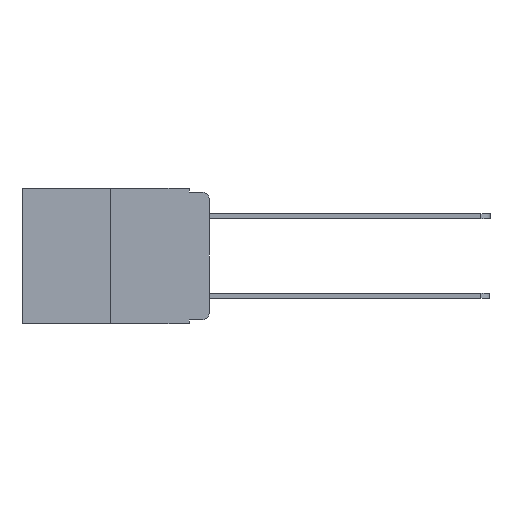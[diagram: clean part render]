
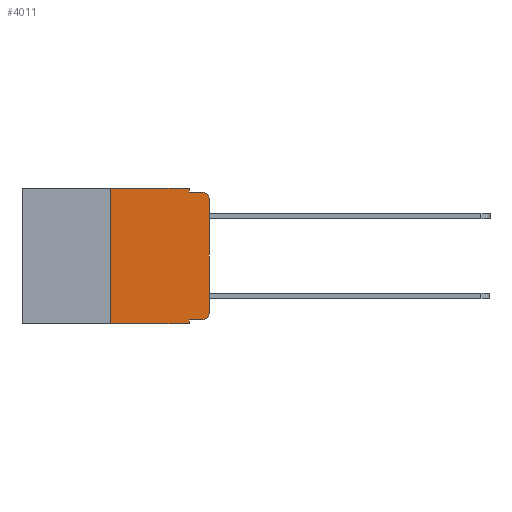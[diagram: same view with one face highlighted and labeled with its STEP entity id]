
A CAD part, left-side view. The second image highlights one B-rep face of the part: STEP entity #4011.
In plain terms, the highlighted planar face has unit normal (-1, 0, 0).
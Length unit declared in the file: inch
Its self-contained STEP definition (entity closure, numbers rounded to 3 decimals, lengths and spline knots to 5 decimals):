
#513 = DIRECTION ( 'NONE',  ( -1., 0., 0. ) ) ;
#564 = LINE ( 'NONE', #9839, #15266 ) ;
#568 = CARTESIAN_POINT ( 'NONE',  ( 0., 0.051, 0. ) ) ;
#686 = LINE ( 'NONE', #568, #10076 ) ;
#818 = VERTEX_POINT ( 'NONE', #4089 ) ;
#826 = DIRECTION ( 'NONE',  ( -1., 0., 0. ) ) ;
#907 = ORIENTED_EDGE ( 'NONE', *, *, #12109, .F. ) ;
#1505 = VERTEX_POINT ( 'NONE', #11846 ) ;
#1702 = VERTEX_POINT ( 'NONE', #4989 ) ;
#1806 = DIRECTION ( 'NONE',  ( 0., 0., -1. ) ) ;
#2162 = CARTESIAN_POINT ( 'NONE',  ( 0., 0.051, -0.343 ) ) ;
#2514 = AXIS2_PLACEMENT_3D ( 'NONE', #7918, #513, #9155 ) ;
#2521 = AXIS2_PLACEMENT_3D ( 'NONE', #10838, #4907, #11024 ) ;
#2619 = ORIENTED_EDGE ( 'NONE', *, *, #12042, .T. ) ;
#3189 = LINE ( 'NONE', #10483, #15379 ) ;
#3351 = VERTEX_POINT ( 'NONE', #6356 ) ;
#3418 = DIRECTION ( 'NONE',  ( 0., -1., 0. ) ) ;
#3820 = ORIENTED_EDGE ( 'NONE', *, *, #11877, .F. ) ;
#3842 = CARTESIAN_POINT ( 'NONE',  ( 0., 0.25, 0. ) ) ;
#3964 = VERTEX_POINT ( 'NONE', #9500 ) ;
#4011 = ADVANCED_FACE ( 'NONE', ( #10536 ), #9906, .F. ) ;
#4089 = CARTESIAN_POINT ( 'NONE',  ( 0., 0., -0.03 ) ) ;
#4232 = ORIENTED_EDGE ( 'NONE', *, *, #5344, .T. ) ;
#4327 = CARTESIAN_POINT ( 'NONE',  ( 0., 0.25, 0. ) ) ;
#4495 = CARTESIAN_POINT ( 'NONE',  ( 0., 0.051, -0.333 ) ) ;
#4907 = DIRECTION ( 'NONE',  ( 1., 0., 0. ) ) ;
#4989 = CARTESIAN_POINT ( 'NONE',  ( 0., 0.051, 0. ) ) ;
#5344 = EDGE_CURVE ( 'NONE', #1505, #5357, #564, .T. ) ;
#5357 = VERTEX_POINT ( 'NONE', #2162 ) ;
#5728 = VECTOR ( 'NONE', #13841, 39.37008 ) ;
#5919 = CARTESIAN_POINT ( 'NONE',  ( 0., 0.051, -0.01 ) ) ;
#6356 = CARTESIAN_POINT ( 'NONE',  ( 0., 0.02, -0.01 ) ) ;
#6676 = CARTESIAN_POINT ( 'NONE',  ( 0., 0.051, -0.01 ) ) ;
#6884 = LINE ( 'NONE', #4327, #12699 ) ;
#6892 = EDGE_LOOP ( 'NONE', ( #14880, #2619, #9582, #9929, #3820, #907, #4232, #7487, #10971, #13953 ) ) ;
#6958 = VERTEX_POINT ( 'NONE', #5919 ) ;
#7487 = ORIENTED_EDGE ( 'NONE', *, *, #12151, .F. ) ;
#7918 = CARTESIAN_POINT ( 'NONE',  ( 0., 0.02, -0.03 ) ) ;
#8233 = CARTESIAN_POINT ( 'NONE',  ( 0., 0.02, -0.313 ) ) ;
#8309 = DIRECTION ( 'NONE',  ( 0., 0., 1. ) ) ;
#8347 = AXIS2_PLACEMENT_3D ( 'NONE', #8233, #826, #9449 ) ;
#8622 = CIRCLE ( 'NONE', #8347, 0.02 ) ;
#8823 = VECTOR ( 'NONE', #10645, 39.37008 ) ;
#9155 = DIRECTION ( 'NONE',  ( 0., 0., -1. ) ) ;
#9190 = LINE ( 'NONE', #15143, #14851 ) ;
#9446 = VERTEX_POINT ( 'NONE', #10137 ) ;
#9449 = DIRECTION ( 'NONE',  ( 0., 0., -1. ) ) ;
#9500 = CARTESIAN_POINT ( 'NONE',  ( 0., 0., -0.313 ) ) ;
#9516 = CARTESIAN_POINT ( 'NONE',  ( 0., 0.473, 0. ) ) ;
#9551 = LINE ( 'NONE', #9516, #8823 ) ;
#9582 = ORIENTED_EDGE ( 'NONE', *, *, #12063, .F. ) ;
#9839 = CARTESIAN_POINT ( 'NONE',  ( 0., 0.473, -0.343 ) ) ;
#9906 = PLANE ( 'NONE',  #2521 ) ;
#9929 = ORIENTED_EDGE ( 'NONE', *, *, #12085, .F. ) ;
#10038 = CARTESIAN_POINT ( 'NONE',  ( 0., 0.051, -0.333 ) ) ;
#10076 = VECTOR ( 'NONE', #1806, 39.37008 ) ;
#10137 = CARTESIAN_POINT ( 'NONE',  ( 0., 0.02, -0.333 ) ) ;
#10483 = CARTESIAN_POINT ( 'NONE',  ( 0., 0.051, 0. ) ) ;
#10536 = FACE_OUTER_BOUND ( 'NONE', #6892, .T. ) ;
#10645 = DIRECTION ( 'NONE',  ( 0., -1., 0. ) ) ;
#10774 = LINE ( 'NONE', #6676, #13376 ) ;
#10838 = CARTESIAN_POINT ( 'NONE',  ( 0., 0.473, 0. ) ) ;
#10971 = ORIENTED_EDGE ( 'NONE', *, *, #12156, .T. ) ;
#11024 = DIRECTION ( 'NONE',  ( 0., 0., -1. ) ) ;
#11594 = DIRECTION ( 'NONE',  ( 0., 0., -1. ) ) ;
#11846 = CARTESIAN_POINT ( 'NONE',  ( 0., 0.25, -0.343 ) ) ;
#11876 = EDGE_CURVE ( 'NONE', #3964, #818, #9190, .T. ) ;
#11877 = EDGE_CURVE ( 'NONE', #13348, #1702, #9551, .T. ) ;
#12042 = EDGE_CURVE ( 'NONE', #818, #3351, #13731, .T. ) ;
#12063 = EDGE_CURVE ( 'NONE', #6958, #3351, #10774, .T. ) ;
#12085 = EDGE_CURVE ( 'NONE', #1702, #6958, #686, .T. ) ;
#12109 = EDGE_CURVE ( 'NONE', #1505, #13348, #6884, .T. ) ;
#12151 = EDGE_CURVE ( 'NONE', #14502, #5357, #3189, .T. ) ;
#12156 = EDGE_CURVE ( 'NONE', #14502, #9446, #15025, .T. ) ;
#12200 = EDGE_CURVE ( 'NONE', #9446, #3964, #8622, .T. ) ;
#12598 = DIRECTION ( 'NONE',  ( 0., 0., 1. ) ) ;
#12699 = VECTOR ( 'NONE', #12598, 39.37008 ) ;
#13348 = VERTEX_POINT ( 'NONE', #3842 ) ;
#13376 = VECTOR ( 'NONE', #14785, 39.37008 ) ;
#13731 = CIRCLE ( 'NONE', #2514, 0.02 ) ;
#13841 = DIRECTION ( 'NONE',  ( 0., -1., 0. ) ) ;
#13953 = ORIENTED_EDGE ( 'NONE', *, *, #12200, .T. ) ;
#14502 = VERTEX_POINT ( 'NONE', #10038 ) ;
#14785 = DIRECTION ( 'NONE',  ( 0., -1., 0. ) ) ;
#14851 = VECTOR ( 'NONE', #8309, 39.37008 ) ;
#14880 = ORIENTED_EDGE ( 'NONE', *, *, #11876, .T. ) ;
#15025 = LINE ( 'NONE', #4495, #5728 ) ;
#15143 = CARTESIAN_POINT ( 'NONE',  ( 0., 0., 0. ) ) ;
#15266 = VECTOR ( 'NONE', #3418, 39.37008 ) ;
#15379 = VECTOR ( 'NONE', #11594, 39.37008 ) ;
